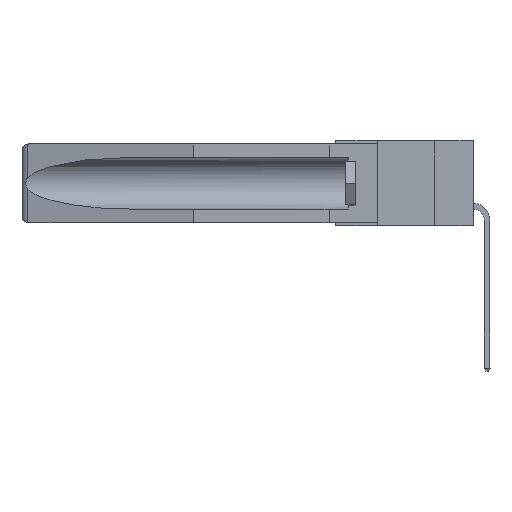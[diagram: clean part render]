
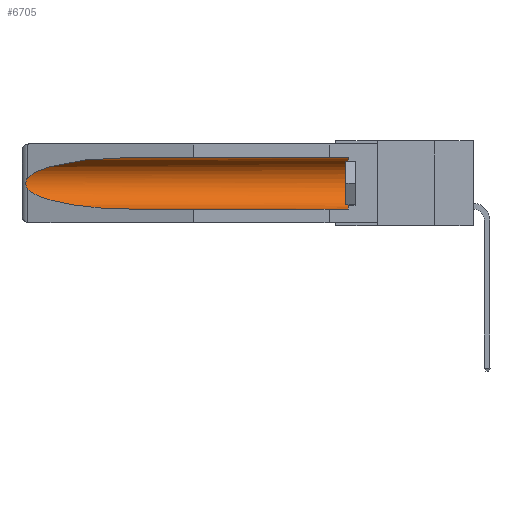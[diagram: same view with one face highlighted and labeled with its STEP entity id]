
A CAD part, left-side view. The second image highlights one B-rep face of the part: STEP entity #6705.
In plain terms, the highlighted cylindrical face has radius 2.857 mm (diameter 5.715 mm), a partial arc.
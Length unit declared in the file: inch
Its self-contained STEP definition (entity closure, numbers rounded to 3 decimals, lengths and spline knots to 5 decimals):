
#370 = VERTEX_POINT ( 'NONE', #2050 ) ;
#612 = AXIS2_PLACEMENT_3D ( 'NONE', #948, #1093, #13423 ) ;
#948 = CARTESIAN_POINT ( 'NONE',  ( 0.155, 0.126, -0.1715 ) ) ;
#1093 = DIRECTION ( 'NONE',  ( 0., -1., 0. ) ) ;
#1261 = CARTESIAN_POINT ( 'NONE',  ( 0.21114, 1.30732, -0.284 ) ) ;
#1629 = DIRECTION ( 'NONE',  ( 0., 1., 0. ) ) ;
#2050 = CARTESIAN_POINT ( 'NONE',  ( 0.26537, 1.52718, -0.14972 ) ) ;
#3027 = ORIENTED_EDGE ( 'NONE', *, *, #4854, .T. ) ;
#3073 = EDGE_LOOP ( 'NONE', ( #3027, #13466, #20803, #17714, #8116, #5082 ) ) ;
#3396 = CARTESIAN_POINT ( 'NONE',  ( 0.155, -0.30754, -0.284 ) ) ;
#3813 = VERTEX_POINT ( 'NONE', #11831 ) ;
#4854 = EDGE_CURVE ( 'NONE', #18909, #370, #5486, .T. ) ;
#5082 = ORIENTED_EDGE ( 'NONE', *, *, #14662, .T. ) ;
#5486 =( BOUNDED_CURVE ( )  B_SPLINE_CURVE ( 3, ( #11011, #14308, #16324, #11090 ),
 .UNSPECIFIED., .F., .F. ) 
 B_SPLINE_CURVE_WITH_KNOTS ( ( 4, 4 ),
 ( 4.71239, 6.08839 ),
 .UNSPECIFIED. ) 
 CURVE ( )  GEOMETRIC_REPRESENTATION_ITEM ( )  RATIONAL_B_SPLINE_CURVE ( ( 1., 0.848, 0.848, 1. ) ) 
 REPRESENTATION_ITEM ( '' )  );
#6423 = EDGE_CURVE ( 'NONE', #370, #3813, #22589, .T. ) ;
#6705 = ADVANCED_FACE ( 'NONE', ( #22831 ), #10687, .F. ) ;
#6955 = CARTESIAN_POINT ( 'NONE',  ( 0.26537, 1.52718, -0.14972 ) ) ;
#6973 = VECTOR ( 'NONE', #1629, 39.37008 ) ;
#7179 =( BOUNDED_CURVE ( )  B_SPLINE_CURVE ( 3, ( #8346, #11907, #1261, #10180 ),
 .UNSPECIFIED., .F., .F. ) 
 B_SPLINE_CURVE_WITH_KNOTS ( ( 4, 4 ),
 ( 0.1948, 1.5708 ),
 .UNSPECIFIED. ) 
 CURVE ( )  GEOMETRIC_REPRESENTATION_ITEM ( )  RATIONAL_B_SPLINE_CURVE ( ( 1., 0.848, 0.848, 1. ) ) 
 REPRESENTATION_ITEM ( '' )  );
#7727 = CARTESIAN_POINT ( 'NONE',  ( 0.155, -0.30754, -0.1715 ) ) ;
#8057 = DIRECTION ( 'NONE',  ( 0., 1., 0. ) ) ;
#8116 = ORIENTED_EDGE ( 'NONE', *, *, #21813, .T. ) ;
#8346 = CARTESIAN_POINT ( 'NONE',  ( 0.26537, 1.52718, -0.19328 ) ) ;
#8739 = CARTESIAN_POINT ( 'NONE',  ( 0.2675, 1.53308, -0.17534 ) ) ;
#8879 = CARTESIAN_POINT ( 'NONE',  ( 0.26537, 1.52718, -0.19328 ) ) ;
#8908 = CARTESIAN_POINT ( 'NONE',  ( 0.155, 1.07973, -0.284 ) ) ;
#9155 = CARTESIAN_POINT ( 'NONE',  ( 0.155, 1.07973, -0.059 ) ) ;
#9274 = DIRECTION ( 'NONE',  ( 0., 0., 1. ) ) ;
#10180 = CARTESIAN_POINT ( 'NONE',  ( 0.155, 1.07973, -0.284 ) ) ;
#10508 = CARTESIAN_POINT ( 'NONE',  ( 0.2673, 1.53269, -0.17917 ) ) ;
#10687 = CYLINDRICAL_SURFACE ( 'NONE', #20511, 0.1125 ) ;
#11011 = CARTESIAN_POINT ( 'NONE',  ( 0.155, 1.07973, -0.059 ) ) ;
#11090 = CARTESIAN_POINT ( 'NONE',  ( 0.26537, 1.52718, -0.14972 ) ) ;
#11554 = CARTESIAN_POINT ( 'NONE',  ( 0.155, -0.30754, -0.059 ) ) ;
#11831 = CARTESIAN_POINT ( 'NONE',  ( 0.26537, 1.52718, -0.19328 ) ) ;
#11894 = LINE ( 'NONE', #11554, #20152 ) ;
#11907 = CARTESIAN_POINT ( 'NONE',  ( 0.25451, 1.48313, -0.24835 ) ) ;
#12312 = CARTESIAN_POINT ( 'NONE',  ( 0.26597, 1.5296, -0.19026 ) ) ;
#12766 = DIRECTION ( 'NONE',  ( 0., 1., 0. ) ) ;
#12799 = LINE ( 'NONE', #3396, #6973 ) ;
#13423 = DIRECTION ( 'NONE',  ( 0., 0., 1. ) ) ;
#13466 = ORIENTED_EDGE ( 'NONE', *, *, #6423, .T. ) ;
#14127 = CARTESIAN_POINT ( 'NONE',  ( 0.2673, 1.5327, -0.16383 ) ) ;
#14308 = CARTESIAN_POINT ( 'NONE',  ( 0.21114, 1.30732, -0.059 ) ) ;
#14662 = EDGE_CURVE ( 'NONE', #17042, #18909, #11894, .T. ) ;
#15331 = EDGE_CURVE ( 'NONE', #17226, #17875, #12799, .T. ) ;
#15748 = CIRCLE ( 'NONE', #612, 0.1125 ) ;
#16324 = CARTESIAN_POINT ( 'NONE',  ( 0.25451, 1.48313, -0.09465 ) ) ;
#17042 = VERTEX_POINT ( 'NONE', #21366 ) ;
#17226 = VERTEX_POINT ( 'NONE', #21897 ) ;
#17714 = ORIENTED_EDGE ( 'NONE', *, *, #15331, .F. ) ;
#17827 = CARTESIAN_POINT ( 'NONE',  ( 0.26597, 1.52961, -0.15275 ) ) ;
#17833 = EDGE_CURVE ( 'NONE', #3813, #17875, #7179, .T. ) ;
#17875 = VERTEX_POINT ( 'NONE', #8908 ) ;
#18909 = VERTEX_POINT ( 'NONE', #9155 ) ;
#19279 = CARTESIAN_POINT ( 'NONE',  ( 0.2675, 1.53308, -0.16763 ) ) ;
#19585 = CARTESIAN_POINT ( 'NONE',  ( 0.26654, 1.53092, -0.15636 ) ) ;
#20152 = VECTOR ( 'NONE', #8057, 39.37008 ) ;
#20511 = AXIS2_PLACEMENT_3D ( 'NONE', #7727, #12766, #9274 ) ;
#20803 = ORIENTED_EDGE ( 'NONE', *, *, #17833, .T. ) ;
#21366 = CARTESIAN_POINT ( 'NONE',  ( 0.155, 0.126, -0.059 ) ) ;
#21813 = EDGE_CURVE ( 'NONE', #17226, #17042, #15748, .T. ) ;
#21897 = CARTESIAN_POINT ( 'NONE',  ( 0.155, 0.126, -0.284 ) ) ;
#22589 = B_SPLINE_CURVE_WITH_KNOTS ( 'NONE', 3,
 ( #6955, #17827, #19585, #14127, #19279, #8739, #10508, #22857, #12312, #8879 ),
 .UNSPECIFIED., .F., .F.,
 ( 4, 2, 2, 2, 4 ),
 ( 0., 0.00029, 0.00058, 0.00087, 0.00117 ),
 .UNSPECIFIED. ) ;
#22831 = FACE_OUTER_BOUND ( 'NONE', #3073, .T. ) ;
#22857 = CARTESIAN_POINT ( 'NONE',  ( 0.26655, 1.53094, -0.18657 ) ) ;
